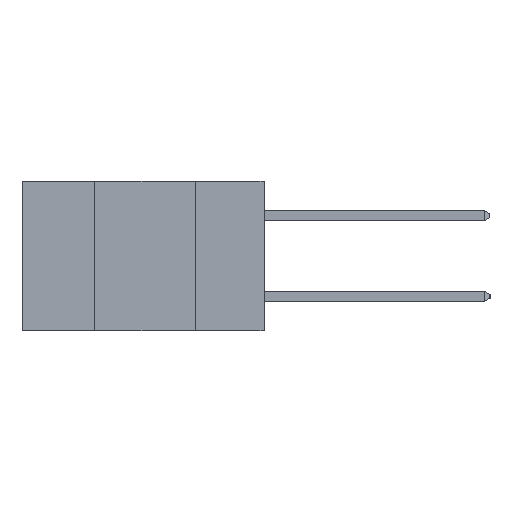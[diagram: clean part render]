
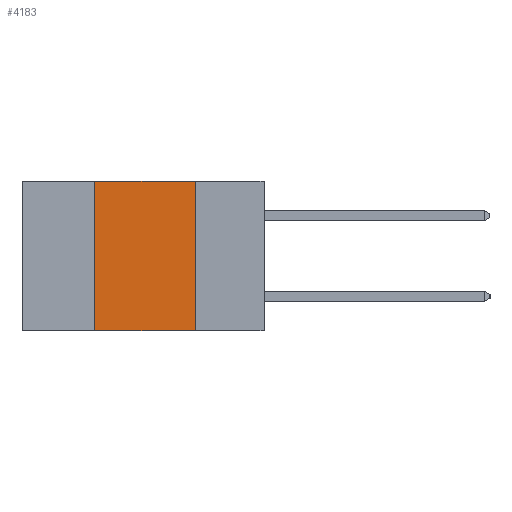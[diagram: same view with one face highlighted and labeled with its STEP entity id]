
A CAD part, left-side view. The second image highlights one B-rep face of the part: STEP entity #4183.
In plain terms, the highlighted planar face has unit normal (-1, 0, 0).
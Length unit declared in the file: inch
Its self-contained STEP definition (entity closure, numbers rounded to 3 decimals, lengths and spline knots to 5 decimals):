
#1688 = CARTESIAN_POINT ( 'NONE',  ( 0., 0.6, -0.37 ) ) ;
#2140 = DIRECTION ( 'NONE',  ( 0., 0., -1. ) ) ;
#2885 = EDGE_LOOP ( 'NONE', ( #14173, #7886, #7805, #3450 ) ) ;
#2980 = CARTESIAN_POINT ( 'NONE',  ( 0., 0.42, -0.37 ) ) ;
#3176 = CARTESIAN_POINT ( 'NONE',  ( 0., 0.6, 0. ) ) ;
#3450 = ORIENTED_EDGE ( 'NONE', *, *, #16157, .T. ) ;
#3467 = VECTOR ( 'NONE', #11763, 39.37008 ) ;
#3936 = LINE ( 'NONE', #3176, #3467 ) ;
#4183 = ADVANCED_FACE ( 'NONE', ( #7703 ), #13847, .F. ) ;
#4816 = LINE ( 'NONE', #1688, #12456 ) ;
#5164 = VERTEX_POINT ( 'NONE', #15127 ) ;
#6808 = CARTESIAN_POINT ( 'NONE',  ( 0., 0.17, -0.37 ) ) ;
#6865 = VERTEX_POINT ( 'NONE', #13161 ) ;
#7584 = VERTEX_POINT ( 'NONE', #6808 ) ;
#7703 = FACE_OUTER_BOUND ( 'NONE', #2885, .T. ) ;
#7805 = ORIENTED_EDGE ( 'NONE', *, *, #18275, .F. ) ;
#7886 = ORIENTED_EDGE ( 'NONE', *, *, #9944, .F. ) ;
#9034 = DIRECTION ( 'NONE',  ( 0., 0., 1. ) ) ;
#9036 = VECTOR ( 'NONE', #9034, 39.37008 ) ;
#9471 = LINE ( 'NONE', #10742, #9939 ) ;
#9854 = VERTEX_POINT ( 'NONE', #2980 ) ;
#9939 = VECTOR ( 'NONE', #2140, 39.37008 ) ;
#9944 = EDGE_CURVE ( 'NONE', #6865, #5164, #3936, .T. ) ;
#10742 = CARTESIAN_POINT ( 'NONE',  ( 0., 0.17, -0.37 ) ) ;
#11482 = EDGE_CURVE ( 'NONE', #5164, #7584, #9471, .T. ) ;
#11763 = DIRECTION ( 'NONE',  ( 0., -1., 0. ) ) ;
#12456 = VECTOR ( 'NONE', #15873, 39.37008 ) ;
#12812 = LINE ( 'NONE', #14611, #9036 ) ;
#13161 = CARTESIAN_POINT ( 'NONE',  ( 0., 0.42, 0. ) ) ;
#13847 = PLANE ( 'NONE',  #17172 ) ;
#14173 = ORIENTED_EDGE ( 'NONE', *, *, #11482, .F. ) ;
#14611 = CARTESIAN_POINT ( 'NONE',  ( 0., 0.42, -0.37 ) ) ;
#15127 = CARTESIAN_POINT ( 'NONE',  ( 0., 0.17, 0. ) ) ;
#15873 = DIRECTION ( 'NONE',  ( 0., -1., 0. ) ) ;
#16157 = EDGE_CURVE ( 'NONE', #9854, #7584, #4816, .T. ) ;
#16938 = DIRECTION ( 'NONE',  ( 0., 0., -1. ) ) ;
#16973 = DIRECTION ( 'NONE',  ( 1., 0., 0. ) ) ;
#17051 = CARTESIAN_POINT ( 'NONE',  ( 0., 0.6, 0. ) ) ;
#17172 = AXIS2_PLACEMENT_3D ( 'NONE', #17051, #16973, #16938 ) ;
#18275 = EDGE_CURVE ( 'NONE', #9854, #6865, #12812, .T. ) ;
